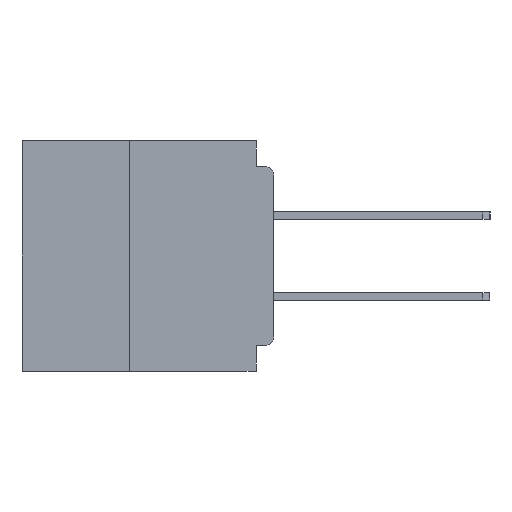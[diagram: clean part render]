
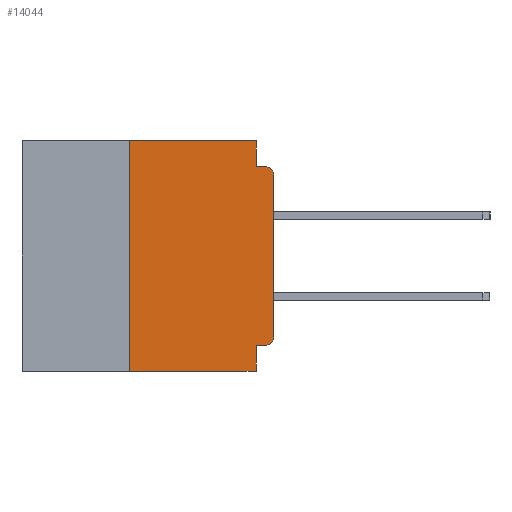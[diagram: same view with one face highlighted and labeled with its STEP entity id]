
A CAD part, left-side view. The second image highlights one B-rep face of the part: STEP entity #14044.
In plain terms, the highlighted planar face has unit normal (-1, 0, 0).
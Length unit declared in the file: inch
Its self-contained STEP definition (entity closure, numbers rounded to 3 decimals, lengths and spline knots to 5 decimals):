
#2 = ORIENTED_EDGE ( 'NONE', *, *, #51888, .F. ) ;
#16 = CARTESIAN_POINT ( 'NONE',  ( 0., 0.437, 0. ) ) ;
#1311 = LINE ( 'NONE', #2165, #35932 ) ;
#2165 = CARTESIAN_POINT ( 'NONE',  ( 0., 0., -0.355 ) ) ;
#2552 = ORIENTED_EDGE ( 'NONE', *, *, #20356, .F. ) ;
#2800 = VECTOR ( 'NONE', #26486, 39.37008 ) ;
#4545 = DIRECTION ( 'NONE',  ( 0., -1., 0. ) ) ;
#5015 = VERTEX_POINT ( 'NONE', #47561 ) ;
#5756 = CIRCLE ( 'NONE', #27908, 0.015 ) ;
#6346 = PLANE ( 'NONE',  #39659 ) ;
#6388 = VECTOR ( 'NONE', #41972, 39.37008 ) ;
#6684 = DIRECTION ( 'NONE',  ( 0., 1., 0. ) ) ;
#7527 = ORIENTED_EDGE ( 'NONE', *, *, #18622, .F. ) ;
#11365 = CARTESIAN_POINT ( 'NONE',  ( 0., 0.015, -0.06 ) ) ;
#11962 = LINE ( 'NONE', #50799, #31803 ) ;
#12634 = LINE ( 'NONE', #36343, #35293 ) ;
#13167 = VERTEX_POINT ( 'NONE', #13708 ) ;
#13708 = CARTESIAN_POINT ( 'NONE',  ( 0., 0.25, -0.4 ) ) ;
#13936 = LINE ( 'NONE', #52086, #38038 ) ;
#14044 = ADVANCED_FACE ( 'NONE', ( #19511 ), #6346, .F. ) ;
#14539 = VERTEX_POINT ( 'NONE', #51311 ) ;
#15376 = CARTESIAN_POINT ( 'NONE',  ( 0., 0.437, 0. ) ) ;
#15616 = DIRECTION ( 'NONE',  ( 0., 0., 1. ) ) ;
#15900 = DIRECTION ( 'NONE',  ( 0., 0., -1. ) ) ;
#17322 = EDGE_LOOP ( 'NONE', ( #27364, #30214, #35890, #2, #2552, #7527, #23005, #24326, #46391, #34783 ) ) ;
#17408 = DIRECTION ( 'NONE',  ( -1., 0., 0. ) ) ;
#17883 = CARTESIAN_POINT ( 'NONE',  ( 0., 0.031, -0.355 ) ) ;
#18373 = VERTEX_POINT ( 'NONE', #25477 ) ;
#18622 = EDGE_CURVE ( 'NONE', #13167, #30223, #12634, .T. ) ;
#19102 = VERTEX_POINT ( 'NONE', #26001 ) ;
#19511 = FACE_OUTER_BOUND ( 'NONE', #17322, .T. ) ;
#19971 = DIRECTION ( 'NONE',  ( 1., 0., 0. ) ) ;
#20356 = EDGE_CURVE ( 'NONE', #30223, #18373, #58152, .T. ) ;
#20388 = CIRCLE ( 'NONE', #34032, 0.015 ) ;
#21927 = CARTESIAN_POINT ( 'NONE',  ( 0., 0.031, 0. ) ) ;
#22927 = EDGE_CURVE ( 'NONE', #28464, #5015, #5756, .T. ) ;
#23005 = ORIENTED_EDGE ( 'NONE', *, *, #24912, .T. ) ;
#23202 = VECTOR ( 'NONE', #25179, 39.37008 ) ;
#23766 = CARTESIAN_POINT ( 'NONE',  ( 0., 0., -0.045 ) ) ;
#24326 = ORIENTED_EDGE ( 'NONE', *, *, #42317, .F. ) ;
#24626 = LINE ( 'NONE', #47715, #23202 ) ;
#24912 = EDGE_CURVE ( 'NONE', #13167, #35847, #13936, .T. ) ;
#25079 = DIRECTION ( 'NONE',  ( 0., -1., 0. ) ) ;
#25179 = DIRECTION ( 'NONE',  ( 0., 0., -1. ) ) ;
#25477 = CARTESIAN_POINT ( 'NONE',  ( 0., 0.031, 0. ) ) ;
#26001 = CARTESIAN_POINT ( 'NONE',  ( 0., 0.031, -0.045 ) ) ;
#26068 = EDGE_CURVE ( 'NONE', #19102, #5015, #55760, .T. ) ;
#26486 = DIRECTION ( 'NONE',  ( 0., 0., -1. ) ) ;
#27364 = ORIENTED_EDGE ( 'NONE', *, *, #57781, .T. ) ;
#27908 = AXIS2_PLACEMENT_3D ( 'NONE', #11365, #43009, #15900 ) ;
#28464 = VERTEX_POINT ( 'NONE', #40962 ) ;
#30214 = ORIENTED_EDGE ( 'NONE', *, *, #22927, .T. ) ;
#30223 = VERTEX_POINT ( 'NONE', #57958 ) ;
#31803 = VECTOR ( 'NONE', #15616, 39.37008 ) ;
#32995 = VERTEX_POINT ( 'NONE', #52459 ) ;
#34032 = AXIS2_PLACEMENT_3D ( 'NONE', #44485, #17408, #49053 ) ;
#34783 = ORIENTED_EDGE ( 'NONE', *, *, #52945, .T. ) ;
#35100 = VERTEX_POINT ( 'NONE', #17883 ) ;
#35293 = VECTOR ( 'NONE', #40884, 39.37008 ) ;
#35847 = VERTEX_POINT ( 'NONE', #55514 ) ;
#35890 = ORIENTED_EDGE ( 'NONE', *, *, #26068, .F. ) ;
#35932 = VECTOR ( 'NONE', #6684, 39.37008 ) ;
#36343 = CARTESIAN_POINT ( 'NONE',  ( 0., 0.25, -0.4 ) ) ;
#38038 = VECTOR ( 'NONE', #25079, 39.37008 ) ;
#38831 = LINE ( 'NONE', #21927, #2800 ) ;
#39659 = AXIS2_PLACEMENT_3D ( 'NONE', #15376, #19971, #51532 ) ;
#40884 = DIRECTION ( 'NONE',  ( 0., 0., 1. ) ) ;
#40962 = CARTESIAN_POINT ( 'NONE',  ( 0., 0., -0.06 ) ) ;
#41972 = DIRECTION ( 'NONE',  ( 0., -1., 0. ) ) ;
#42317 = EDGE_CURVE ( 'NONE', #35100, #35847, #24626, .T. ) ;
#43009 = DIRECTION ( 'NONE',  ( -1., 0., 0. ) ) ;
#44485 = CARTESIAN_POINT ( 'NONE',  ( 0., 0.015, -0.34 ) ) ;
#44849 = VECTOR ( 'NONE', #4545, 39.37008 ) ;
#46068 = EDGE_CURVE ( 'NONE', #32995, #35100, #1311, .T. ) ;
#46391 = ORIENTED_EDGE ( 'NONE', *, *, #46068, .F. ) ;
#47561 = CARTESIAN_POINT ( 'NONE',  ( 0., 0.015, -0.045 ) ) ;
#47715 = CARTESIAN_POINT ( 'NONE',  ( 0., 0.031, -0.4 ) ) ;
#49053 = DIRECTION ( 'NONE',  ( 0., 0., -1. ) ) ;
#50799 = CARTESIAN_POINT ( 'NONE',  ( 0., 0., 0. ) ) ;
#51311 = CARTESIAN_POINT ( 'NONE',  ( 0., 0., -0.34 ) ) ;
#51532 = DIRECTION ( 'NONE',  ( 0., 0., -1. ) ) ;
#51888 = EDGE_CURVE ( 'NONE', #18373, #19102, #38831, .T. ) ;
#52086 = CARTESIAN_POINT ( 'NONE',  ( 0., 0.437, -0.4 ) ) ;
#52459 = CARTESIAN_POINT ( 'NONE',  ( 0., 0.015, -0.355 ) ) ;
#52945 = EDGE_CURVE ( 'NONE', #32995, #14539, #20388, .T. ) ;
#55514 = CARTESIAN_POINT ( 'NONE',  ( 0., 0.031, -0.4 ) ) ;
#55760 = LINE ( 'NONE', #23766, #6388 ) ;
#57781 = EDGE_CURVE ( 'NONE', #14539, #28464, #11962, .T. ) ;
#57958 = CARTESIAN_POINT ( 'NONE',  ( 0., 0.25, 0. ) ) ;
#58152 = LINE ( 'NONE', #16, #44849 ) ;
